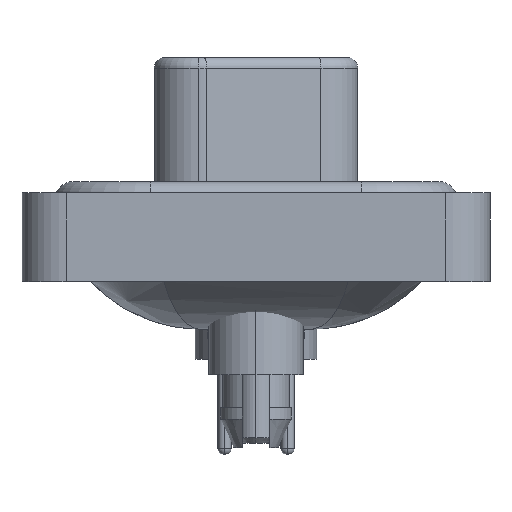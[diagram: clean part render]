
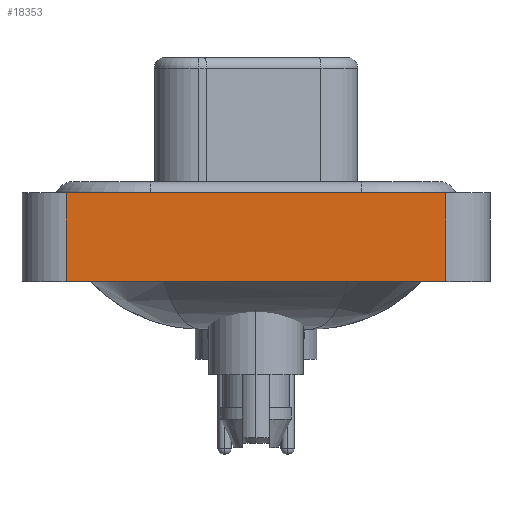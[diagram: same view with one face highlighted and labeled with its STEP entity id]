
A CAD part, left-side view. The second image highlights one B-rep face of the part: STEP entity #18353.
In plain terms, the highlighted planar face has unit normal (-1, 0, 0).
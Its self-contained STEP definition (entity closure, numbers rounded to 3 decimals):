
#266 = FACE_OUTER_BOUND ( 'NONE', #19055, .T. ) ;
#2353 = CARTESIAN_POINT ( 'NONE',  ( -7.3, -8.55, -3.6 ) ) ;
#2730 = VERTEX_POINT ( 'NONE', #11390 ) ;
#3823 = VECTOR ( 'NONE', #25250, 1000. ) ;
#3928 = CARTESIAN_POINT ( 'NONE',  ( -7.3, 8.55, -3.6 ) ) ;
#4000 = VERTEX_POINT ( 'NONE', #11551 ) ;
#4653 = ORIENTED_EDGE ( 'NONE', *, *, #18489, .F. ) ;
#4698 = LINE ( 'NONE', #10570, #19792 ) ;
#5719 = CARTESIAN_POINT ( 'NONE',  ( -7.3, 8.55, -3.6 ) ) ;
#6729 = VERTEX_POINT ( 'NONE', #18299 ) ;
#6897 = DIRECTION ( 'NONE',  ( 0., 0., 1. ) ) ;
#8218 = DIRECTION ( 'NONE',  ( 0., 0., 1. ) ) ;
#8291 = LINE ( 'NONE', #13895, #16286 ) ;
#8361 = VERTEX_POINT ( 'NONE', #5719 ) ;
#10570 = CARTESIAN_POINT ( 'NONE',  ( -7.3, -8.55, 0.4 ) ) ;
#11390 = CARTESIAN_POINT ( 'NONE',  ( -7.3, 8.55, 0.4 ) ) ;
#11551 = CARTESIAN_POINT ( 'NONE',  ( -7.3, -8.55, -3.6 ) ) ;
#13895 = CARTESIAN_POINT ( 'NONE',  ( -7.3, -8.55, -3.6 ) ) ;
#15649 = LINE ( 'NONE', #3928, #3823 ) ;
#15983 = DIRECTION ( 'NONE',  ( 0., -1., 0. ) ) ;
#16286 = VECTOR ( 'NONE', #15983, 1000. ) ;
#16293 = DIRECTION ( 'NONE',  ( -1., 0., 0. ) ) ;
#17080 = ORIENTED_EDGE ( 'NONE', *, *, #17168, .F. ) ;
#17168 = EDGE_CURVE ( 'NONE', #8361, #2730, #15649, .T. ) ;
#18299 = CARTESIAN_POINT ( 'NONE',  ( -7.3, -8.55, 0.4 ) ) ;
#18353 = ADVANCED_FACE ( 'NONE', ( #266 ), #24210, .T. ) ;
#18389 = DIRECTION ( 'NONE',  ( 0., -1., 0. ) ) ;
#18489 = EDGE_CURVE ( 'NONE', #2730, #6729, #4698, .T. ) ;
#19055 = EDGE_LOOP ( 'NONE', ( #21992, #4653, #17080, #22805 ) ) ;
#19768 = EDGE_CURVE ( 'NONE', #4000, #6729, #20979, .T. ) ;
#19792 = VECTOR ( 'NONE', #18389, 1000. ) ;
#20979 = LINE ( 'NONE', #24733, #25042 ) ;
#21992 = ORIENTED_EDGE ( 'NONE', *, *, #19768, .T. ) ;
#22805 = ORIENTED_EDGE ( 'NONE', *, *, #23341, .T. ) ;
#23341 = EDGE_CURVE ( 'NONE', #8361, #4000, #8291, .T. ) ;
#24210 = PLANE ( 'NONE',  #24342 ) ;
#24342 = AXIS2_PLACEMENT_3D ( 'NONE', #2353, #16293, #8218 ) ;
#24733 = CARTESIAN_POINT ( 'NONE',  ( -7.3, -8.55, -3.6 ) ) ;
#25042 = VECTOR ( 'NONE', #6897, 1000. ) ;
#25250 = DIRECTION ( 'NONE',  ( 0., 0., 1. ) ) ;
